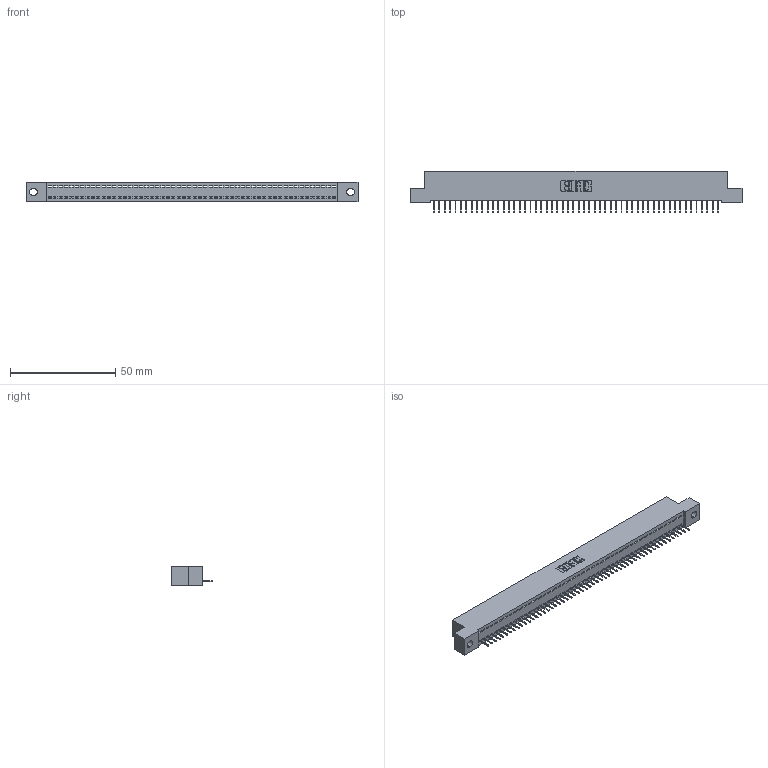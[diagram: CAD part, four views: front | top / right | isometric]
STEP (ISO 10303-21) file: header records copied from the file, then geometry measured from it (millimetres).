
FILE_DESCRIPTION (( 'STEP AP203' ), '1' );
FILE_NAME ('392-054-524-102.STEP', '2018-08-17T08:39:15', ( '' ), ( '' ), 'SwSTEP 2.0', 'SolidWorks 2016', '' );
FILE_SCHEMA (( 'CONFIG_CONTROL_DESIGN' ));
Length unit declared in the file: inch
Products named in the file (3): 342 Part_.128 Slot; 345-292-001_345-293-124; 392-054-524-102
Assembly tree (55 placements, depth 2):
  392-054-524-102
    342 Part_.128 Slot
    345-292-001_345-293-124  x54
Bounding box: 157.48 x 19.69 x 9.4 mm (x, y, z)
Volume: 13586.6 mm3; surface area: 19272.4 mm2
Topology: 55 solids, 55 shells, 3462 faces, 10031 edges, 6470 vertices
Faces by surface type: plane 2662, cylinder 800
Entity records: 31537 total; most frequent: CARTESIAN_POINT 5444, ORIENTED_EDGE 5434, DIRECTION 4569, EDGE_CURVE 2717, LINE 2593, VECTOR 2593, VERTEX_POINT 1806, AXIS2_PLACEMENT_3D 988
